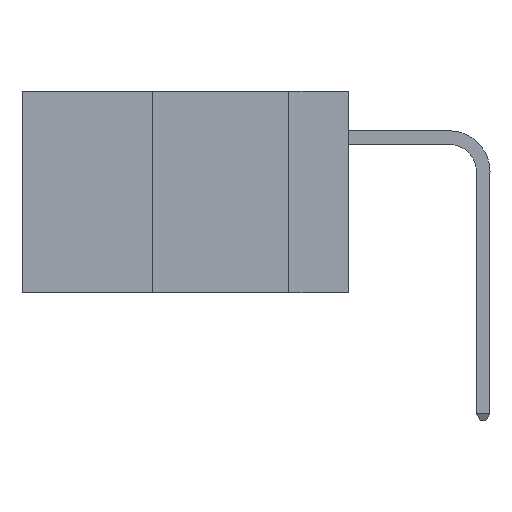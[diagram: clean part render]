
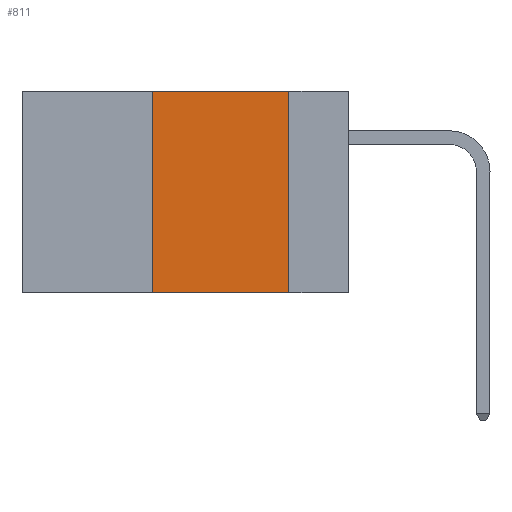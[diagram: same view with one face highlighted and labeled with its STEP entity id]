
A CAD part, left-side view. The second image highlights one B-rep face of the part: STEP entity #811.
In plain terms, the highlighted planar face has unit normal (-1, 0, 0).
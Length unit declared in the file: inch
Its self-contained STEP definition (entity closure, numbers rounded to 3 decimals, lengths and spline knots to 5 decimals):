
#61 = VECTOR ( 'NONE', #4405, 39.37008 ) ;
#540 = EDGE_CURVE ( 'NONE', #9291, #3719, #4947, .T. ) ;
#811 = ADVANCED_FACE ( 'NONE', ( #8802 ), #6873, .F. ) ;
#891 = LINE ( 'NONE', #15176, #61 ) ;
#967 = EDGE_LOOP ( 'NONE', ( #1025, #2670, #1537, #12261 ) ) ;
#1025 = ORIENTED_EDGE ( 'NONE', *, *, #15432, .F. ) ;
#1537 = ORIENTED_EDGE ( 'NONE', *, *, #540, .F. ) ;
#2108 = VECTOR ( 'NONE', #5174, 39.37008 ) ;
#2670 = ORIENTED_EDGE ( 'NONE', *, *, #8812, .F. ) ;
#3288 = DIRECTION ( 'NONE',  ( 0., -1., 0. ) ) ;
#3719 = VERTEX_POINT ( 'NONE', #15344 ) ;
#3966 = CARTESIAN_POINT ( 'NONE',  ( 0., 0.11, -0.37 ) ) ;
#4386 = CARTESIAN_POINT ( 'NONE',  ( 0., 0.6, 0. ) ) ;
#4405 = DIRECTION ( 'NONE',  ( 0., 0., -1. ) ) ;
#4947 = LINE ( 'NONE', #16391, #14378 ) ;
#5174 = DIRECTION ( 'NONE',  ( 0., -1., 0. ) ) ;
#5626 = DIRECTION ( 'NONE',  ( 0., 0., -1. ) ) ;
#5711 = LINE ( 'NONE', #10854, #2108 ) ;
#5913 = CARTESIAN_POINT ( 'NONE',  ( 0., 0.6, -0.37 ) ) ;
#6873 = PLANE ( 'NONE',  #16309 ) ;
#8802 = FACE_OUTER_BOUND ( 'NONE', #967, .T. ) ;
#8812 = EDGE_CURVE ( 'NONE', #3719, #14209, #5711, .T. ) ;
#9291 = VERTEX_POINT ( 'NONE', #15888 ) ;
#10854 = CARTESIAN_POINT ( 'NONE',  ( 0., 0.6, 0. ) ) ;
#11057 = DIRECTION ( 'NONE',  ( 1., 0., 0. ) ) ;
#11071 = VECTOR ( 'NONE', #3288, 39.37008 ) ;
#11774 = VERTEX_POINT ( 'NONE', #3966 ) ;
#12261 = ORIENTED_EDGE ( 'NONE', *, *, #15476, .T. ) ;
#14209 = VERTEX_POINT ( 'NONE', #17212 ) ;
#14378 = VECTOR ( 'NONE', #15169, 39.37008 ) ;
#14478 = LINE ( 'NONE', #5913, #11071 ) ;
#15169 = DIRECTION ( 'NONE',  ( 0., 0., 1. ) ) ;
#15176 = CARTESIAN_POINT ( 'NONE',  ( 0., 0.11, 0. ) ) ;
#15344 = CARTESIAN_POINT ( 'NONE',  ( 0., 0.36, 0. ) ) ;
#15432 = EDGE_CURVE ( 'NONE', #14209, #11774, #891, .T. ) ;
#15476 = EDGE_CURVE ( 'NONE', #9291, #11774, #14478, .T. ) ;
#15888 = CARTESIAN_POINT ( 'NONE',  ( 0., 0.36, -0.37 ) ) ;
#16309 = AXIS2_PLACEMENT_3D ( 'NONE', #4386, #11057, #5626 ) ;
#16391 = CARTESIAN_POINT ( 'NONE',  ( 0., 0.36, 0. ) ) ;
#17212 = CARTESIAN_POINT ( 'NONE',  ( 0., 0.11, 0. ) ) ;
